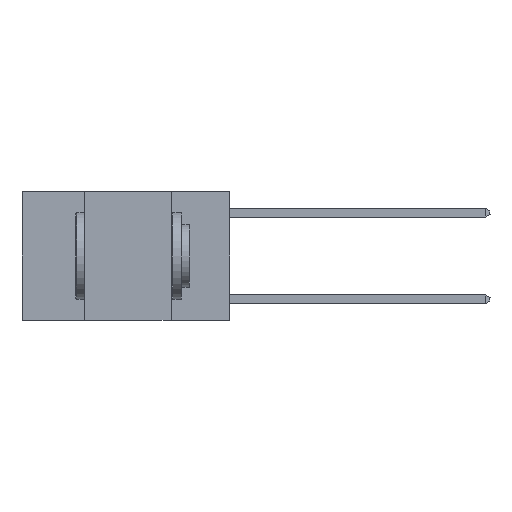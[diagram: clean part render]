
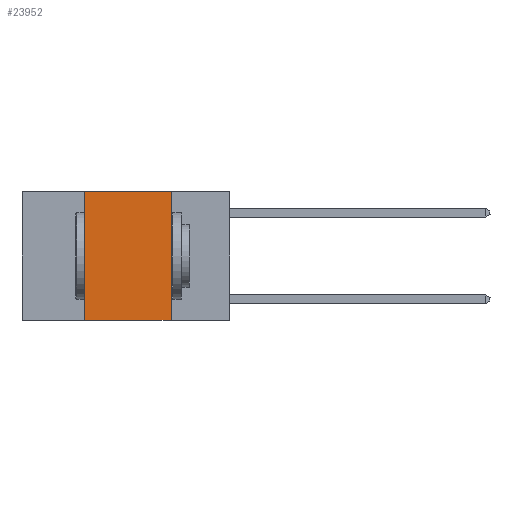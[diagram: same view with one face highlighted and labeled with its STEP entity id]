
A CAD part, left-side view. The second image highlights one B-rep face of the part: STEP entity #23952.
In plain terms, the highlighted planar face has unit normal (-1, 0, 0).
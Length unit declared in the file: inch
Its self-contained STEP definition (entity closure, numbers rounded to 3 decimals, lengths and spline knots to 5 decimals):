
#35 = PLANE ( 'NONE',  #11349 ) ;
#244 = EDGE_CURVE ( 'NONE', #16360, #9270, #3229, .T. ) ;
#655 = ORIENTED_EDGE ( 'NONE', *, *, #3378, .F. ) ;
#1473 = VECTOR ( 'NONE', #11928, 39.37008 ) ;
#2505 = CARTESIAN_POINT ( 'NONE',  ( 0., 0.42, 0. ) ) ;
#3229 = LINE ( 'NONE', #3601, #23143 ) ;
#3378 = EDGE_CURVE ( 'NONE', #20676, #22638, #15766, .T. ) ;
#3601 = CARTESIAN_POINT ( 'NONE',  ( 0., 0.17, 0. ) ) ;
#4631 = EDGE_LOOP ( 'NONE', ( #5424, #5107, #655, #12558 ) ) ;
#5107 = ORIENTED_EDGE ( 'NONE', *, *, #11437, .F. ) ;
#5268 = CARTESIAN_POINT ( 'NONE',  ( 0., 0.6, -0.37 ) ) ;
#5424 = ORIENTED_EDGE ( 'NONE', *, *, #244, .F. ) ;
#5657 = DIRECTION ( 'NONE',  ( 1., 0., 0. ) ) ;
#8224 = LINE ( 'NONE', #10430, #21407 ) ;
#9032 = EDGE_CURVE ( 'NONE', #20676, #9270, #12805, .T. ) ;
#9270 = VERTEX_POINT ( 'NONE', #10172 ) ;
#10172 = CARTESIAN_POINT ( 'NONE',  ( 0., 0.17, -0.37 ) ) ;
#10430 = CARTESIAN_POINT ( 'NONE',  ( 0., 0.6, 0. ) ) ;
#10765 = DIRECTION ( 'NONE',  ( 0., 0., -1. ) ) ;
#11349 = AXIS2_PLACEMENT_3D ( 'NONE', #20365, #5657, #18872 ) ;
#11437 = EDGE_CURVE ( 'NONE', #22638, #16360, #8224, .T. ) ;
#11928 = DIRECTION ( 'NONE',  ( 0., 0., 1. ) ) ;
#12558 = ORIENTED_EDGE ( 'NONE', *, *, #9032, .T. ) ;
#12805 = LINE ( 'NONE', #5268, #22764 ) ;
#15348 = CARTESIAN_POINT ( 'NONE',  ( 0., 0.42, 0. ) ) ;
#15766 = LINE ( 'NONE', #2505, #1473 ) ;
#16360 = VERTEX_POINT ( 'NONE', #16705 ) ;
#16705 = CARTESIAN_POINT ( 'NONE',  ( 0., 0.17, 0. ) ) ;
#18872 = DIRECTION ( 'NONE',  ( 0., 0., -1. ) ) ;
#20365 = CARTESIAN_POINT ( 'NONE',  ( 0., 0.6, 0. ) ) ;
#20676 = VERTEX_POINT ( 'NONE', #24206 ) ;
#21407 = VECTOR ( 'NONE', #23846, 39.37008 ) ;
#22100 = DIRECTION ( 'NONE',  ( 0., -1., 0. ) ) ;
#22619 = FACE_OUTER_BOUND ( 'NONE', #4631, .T. ) ;
#22638 = VERTEX_POINT ( 'NONE', #15348 ) ;
#22764 = VECTOR ( 'NONE', #22100, 39.37008 ) ;
#23143 = VECTOR ( 'NONE', #10765, 39.37008 ) ;
#23846 = DIRECTION ( 'NONE',  ( 0., -1., 0. ) ) ;
#23952 = ADVANCED_FACE ( 'NONE', ( #22619 ), #35, .F. ) ;
#24206 = CARTESIAN_POINT ( 'NONE',  ( 0., 0.42, -0.37 ) ) ;
